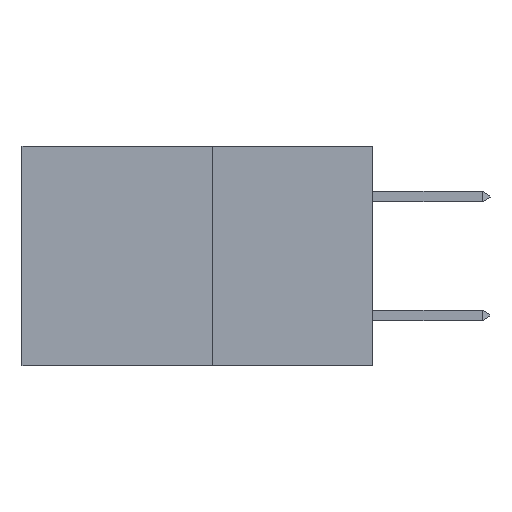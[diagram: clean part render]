
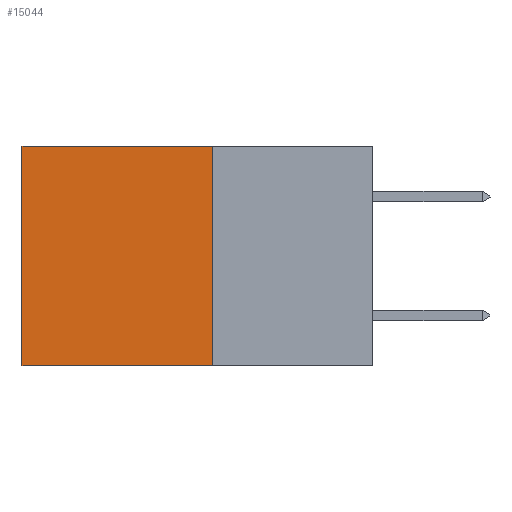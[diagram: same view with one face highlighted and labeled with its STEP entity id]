
A CAD part, left-side view. The second image highlights one B-rep face of the part: STEP entity #15044.
In plain terms, the highlighted planar face has unit normal (-1, 0, 0).
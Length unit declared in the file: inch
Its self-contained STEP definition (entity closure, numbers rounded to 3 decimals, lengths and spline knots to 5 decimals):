
#658 = ORIENTED_EDGE ( 'NONE', *, *, #7481, .T. ) ;
#710 = CARTESIAN_POINT ( 'NONE',  ( 0.277, 0.59, 0. ) ) ;
#951 = CARTESIAN_POINT ( 'NONE',  ( 0.277, 0.27, -0.37 ) ) ;
#2017 = FACE_OUTER_BOUND ( 'NONE', #9135, .T. ) ;
#2806 = VECTOR ( 'NONE', #4806, 39.37008 ) ;
#4145 = VERTEX_POINT ( 'NONE', #710 ) ;
#4806 = DIRECTION ( 'NONE',  ( 0., 0., -1. ) ) ;
#4903 = CARTESIAN_POINT ( 'NONE',  ( 0.277, 0.59, -0.37 ) ) ;
#5063 = CARTESIAN_POINT ( 'NONE',  ( 0.277, 0.27, -0.37 ) ) ;
#5461 = CARTESIAN_POINT ( 'NONE',  ( 0.277, 0.27, 0. ) ) ;
#6071 = ORIENTED_EDGE ( 'NONE', *, *, #7338, .F. ) ;
#6109 = ORIENTED_EDGE ( 'NONE', *, *, #12716, .T. ) ;
#6121 = CARTESIAN_POINT ( 'NONE',  ( 0.277, 0.27, -0.37 ) ) ;
#6218 = DIRECTION ( 'NONE',  ( 0., 0., -1. ) ) ;
#6597 = LINE ( 'NONE', #9079, #14119 ) ;
#6659 = CARTESIAN_POINT ( 'NONE',  ( 0.277, 0.27, -0.37 ) ) ;
#6673 = DIRECTION ( 'NONE',  ( 0., 1., 0. ) ) ;
#6793 = LINE ( 'NONE', #6659, #10559 ) ;
#7038 = LINE ( 'NONE', #4903, #2806 ) ;
#7281 = EDGE_CURVE ( 'NONE', #17863, #16654, #6793, .T. ) ;
#7338 = EDGE_CURVE ( 'NONE', #8784, #17863, #17885, .T. ) ;
#7419 = PLANE ( 'NONE',  #10565 ) ;
#7481 = EDGE_CURVE ( 'NONE', #4145, #16654, #7038, .T. ) ;
#8784 = VERTEX_POINT ( 'NONE', #5461 ) ;
#9036 = DIRECTION ( 'NONE',  ( 0., 0., -1. ) ) ;
#9079 = CARTESIAN_POINT ( 'NONE',  ( 0.277, 0.27, 0. ) ) ;
#9135 = EDGE_LOOP ( 'NONE', ( #658, #20329, #6071, #6109 ) ) ;
#9583 = VECTOR ( 'NONE', #6218, 39.37008 ) ;
#9840 = CARTESIAN_POINT ( 'NONE',  ( 0.277, 0.59, -0.37 ) ) ;
#10559 = VECTOR ( 'NONE', #6673, 39.37008 ) ;
#10565 = AXIS2_PLACEMENT_3D ( 'NONE', #951, #18398, #9036 ) ;
#12283 = DIRECTION ( 'NONE',  ( 0., 1., 0. ) ) ;
#12716 = EDGE_CURVE ( 'NONE', #8784, #4145, #6597, .T. ) ;
#14119 = VECTOR ( 'NONE', #12283, 39.37008 ) ;
#15044 = ADVANCED_FACE ( 'NONE', ( #2017 ), #7419, .F. ) ;
#16654 = VERTEX_POINT ( 'NONE', #9840 ) ;
#17863 = VERTEX_POINT ( 'NONE', #5063 ) ;
#17885 = LINE ( 'NONE', #6121, #9583 ) ;
#18398 = DIRECTION ( 'NONE',  ( 1., 0., 0. ) ) ;
#20329 = ORIENTED_EDGE ( 'NONE', *, *, #7281, .F. ) ;
